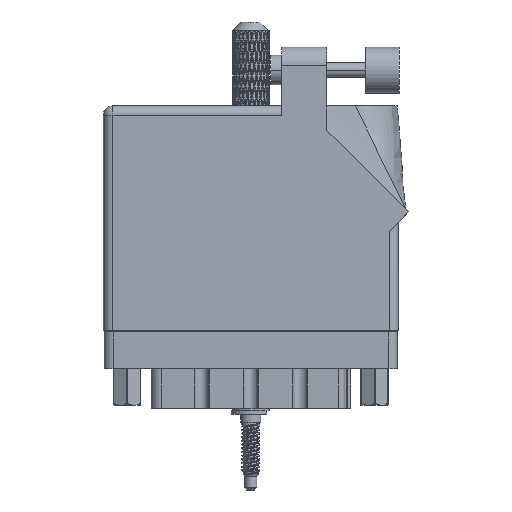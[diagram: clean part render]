
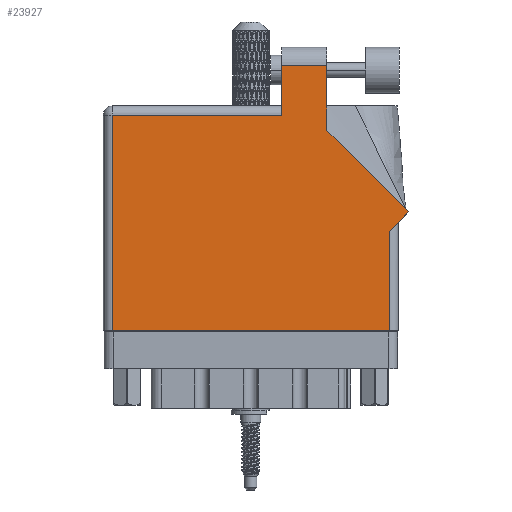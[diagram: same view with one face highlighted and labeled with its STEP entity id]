
A CAD part, front view. The second image highlights one B-rep face of the part: STEP entity #23927.
In plain terms, the highlighted face is planar.
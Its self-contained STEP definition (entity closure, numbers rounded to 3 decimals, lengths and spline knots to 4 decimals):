
#4115 = CARTESIAN_POINT ( 'NONE',  ( 0.062, 0., 0. ) ) ;
#7693 = DIRECTION ( 'NONE',  ( 0.707, 0.707, 0. ) ) ;
#9088 = CARTESIAN_POINT ( 'NONE',  ( 1.217, 1.468, 0. ) ) ;
#12681 = VECTOR ( 'NONE', #16039, 39.3701 ) ;
#16039 = DIRECTION ( 'NONE',  ( 0., -1., 0. ) ) ;
#19088 = CARTESIAN_POINT ( 'NONE',  ( 1.524, 1.805, 0. ) ) ;
#19831 = EDGE_CURVE ( 'NONE', #70581, #74274, #22007, .T. ) ;
#20677 = VERTEX_POINT ( 'NONE', #53654 ) ;
#21356 = ORIENTED_EDGE ( 'NONE', *, *, #68850, .T. ) ;
#21371 = VERTEX_POINT ( 'NONE', #4115 ) ;
#22007 = LINE ( 'NONE', #87588, #112883 ) ;
#23927 = ADVANCED_FACE ( 'NONE', ( #27194 ), #44599, .F. ) ;
#25111 = VERTEX_POINT ( 'NONE', #26538 ) ;
#25688 = DIRECTION ( 'NONE',  ( 0., -1., 0. ) ) ;
#26052 = EDGE_CURVE ( 'NONE', #20677, #21371, #81074, .T. ) ;
#26538 = CARTESIAN_POINT ( 'NONE',  ( 1.217, 1.805, 0. ) ) ;
#27194 = FACE_OUTER_BOUND ( 'NONE', #42829, .T. ) ;
#30219 = LINE ( 'NONE', #64393, #98699 ) ;
#30364 = ORIENTED_EDGE ( 'NONE', *, *, #54560, .T. ) ;
#33185 = CARTESIAN_POINT ( 'NONE',  ( 0.062, 0., 0. ) ) ;
#34801 = VERTEX_POINT ( 'NONE', #19088 ) ;
#37132 = ORIENTED_EDGE ( 'NONE', *, *, #19831, .T. ) ;
#37137 = DIRECTION ( 'NONE',  ( -1., 0., 0. ) ) ;
#37779 = VECTOR ( 'NONE', #53767, 39.3701 ) ;
#40164 = VECTOR ( 'NONE', #112540, 39.3701 ) ;
#41854 = ORIENTED_EDGE ( 'NONE', *, *, #77270, .T. ) ;
#42829 = EDGE_LOOP ( 'NONE', ( #30364, #93149, #21356, #41854, #112232, #92370, #37132, #102321, #56835 ) ) ;
#43007 = EDGE_CURVE ( 'NONE', #21371, #70581, #115737, .T. ) ;
#44147 = CARTESIAN_POINT ( 'NONE',  ( 1.948, 0.675, 0. ) ) ;
#44599 = PLANE ( 'NONE',  #85605 ) ;
#45649 = CARTESIAN_POINT ( 'NONE',  ( 2.0807, 0.8077, 0. ) ) ;
#46348 = CARTESIAN_POINT ( 'NONE',  ( 1.217, 1.805, 0. ) ) ;
#47483 = EDGE_CURVE ( 'NONE', #67672, #75443, #30219, .T. ) ;
#48698 = VECTOR ( 'NONE', #115773, 39.3701 ) ;
#48868 = VECTOR ( 'NONE', #25688, 39.3701 ) ;
#50466 = CARTESIAN_POINT ( 'NONE',  ( 1.524, 1.3644, 0. ) ) ;
#53654 = CARTESIAN_POINT ( 'NONE',  ( 0.062, 1.468, 0. ) ) ;
#53767 = DIRECTION ( 'NONE',  ( -1., 0., 0. ) ) ;
#54560 = EDGE_CURVE ( 'NONE', #75443, #34801, #79254, .T. ) ;
#54748 = VERTEX_POINT ( 'NONE', #9088 ) ;
#55083 = CARTESIAN_POINT ( 'NONE',  ( 0., 1.53, 0. ) ) ;
#56835 = ORIENTED_EDGE ( 'NONE', *, *, #47483, .T. ) ;
#57384 = EDGE_CURVE ( 'NONE', #74274, #67672, #74557, .T. ) ;
#58037 = CARTESIAN_POINT ( 'NONE',  ( 1.948, 0., 0. ) ) ;
#58737 = LINE ( 'NONE', #80692, #100652 ) ;
#59417 = CARTESIAN_POINT ( 'NONE',  ( 1.524, 1.3644, 0. ) ) ;
#61078 = CARTESIAN_POINT ( 'NONE',  ( 2.01, 0.737, 0. ) ) ;
#61515 = LINE ( 'NONE', #46348, #37779 ) ;
#64393 = CARTESIAN_POINT ( 'NONE',  ( 2.0807, 0.8077, 0. ) ) ;
#67672 = VERTEX_POINT ( 'NONE', #45649 ) ;
#68083 = DIRECTION ( 'NONE',  ( 0., 1., 0. ) ) ;
#68850 = EDGE_CURVE ( 'NONE', #25111, #54748, #107594, .T. ) ;
#70176 = CARTESIAN_POINT ( 'NONE',  ( 1.217, 1.53, 0. ) ) ;
#70581 = VERTEX_POINT ( 'NONE', #58037 ) ;
#74274 = VERTEX_POINT ( 'NONE', #44147 ) ;
#74557 = LINE ( 'NONE', #61078, #110843 ) ;
#75443 = VERTEX_POINT ( 'NONE', #50466 ) ;
#77270 = EDGE_CURVE ( 'NONE', #54748, #20677, #58737, .T. ) ;
#77380 = EDGE_CURVE ( 'NONE', #34801, #25111, #61515, .T. ) ;
#78299 = CARTESIAN_POINT ( 'NONE',  ( 0., 0., 0. ) ) ;
#79254 = LINE ( 'NONE', #59417, #40164 ) ;
#80692 = CARTESIAN_POINT ( 'NONE',  ( 0., 1.468, 0. ) ) ;
#81074 = LINE ( 'NONE', #33185, #12681 ) ;
#85605 = AXIS2_PLACEMENT_3D ( 'NONE', #55083, #90689, #37137 ) ;
#87588 = CARTESIAN_POINT ( 'NONE',  ( 1.948, 0.737, 0. ) ) ;
#90600 = DIRECTION ( 'NONE',  ( -0.707, 0.707, 0. ) ) ;
#90689 = DIRECTION ( 'NONE',  ( 0., 0., -1. ) ) ;
#92370 = ORIENTED_EDGE ( 'NONE', *, *, #43007, .T. ) ;
#93149 = ORIENTED_EDGE ( 'NONE', *, *, #77380, .T. ) ;
#98699 = VECTOR ( 'NONE', #90600, 39.3701 ) ;
#99463 = DIRECTION ( 'NONE',  ( -1., 0., 0. ) ) ;
#100652 = VECTOR ( 'NONE', #99463, 39.3701 ) ;
#102321 = ORIENTED_EDGE ( 'NONE', *, *, #57384, .T. ) ;
#107594 = LINE ( 'NONE', #70176, #48868 ) ;
#110843 = VECTOR ( 'NONE', #7693, 39.3701 ) ;
#112232 = ORIENTED_EDGE ( 'NONE', *, *, #26052, .T. ) ;
#112540 = DIRECTION ( 'NONE',  ( 0., 1., 0. ) ) ;
#112883 = VECTOR ( 'NONE', #68083, 39.3701 ) ;
#115737 = LINE ( 'NONE', #78299, #48698 ) ;
#115773 = DIRECTION ( 'NONE',  ( 1., 0., 0. ) ) ;
